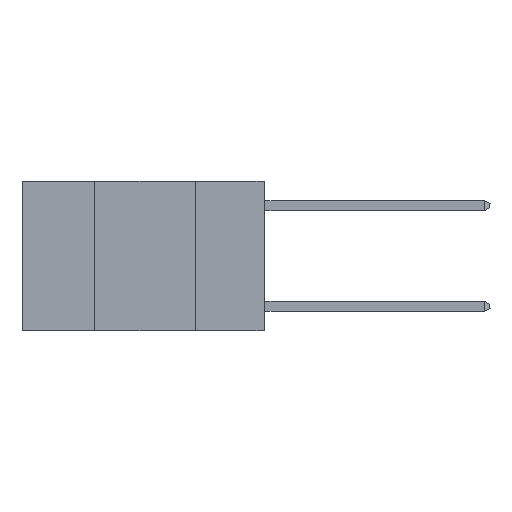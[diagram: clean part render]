
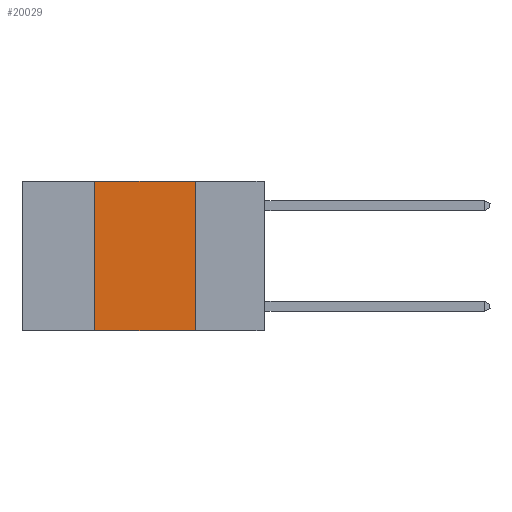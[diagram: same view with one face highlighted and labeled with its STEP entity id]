
A CAD part, left-side view. The second image highlights one B-rep face of the part: STEP entity #20029.
In plain terms, the highlighted planar face has unit normal (-1, 0, 0).
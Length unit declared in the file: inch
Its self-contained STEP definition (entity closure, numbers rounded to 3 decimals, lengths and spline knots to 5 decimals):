
#322 = DIRECTION ( 'NONE',  ( 0., 0., -1. ) ) ;
#1117 = DIRECTION ( 'NONE',  ( 0., 0., 1. ) ) ;
#1171 = ORIENTED_EDGE ( 'NONE', *, *, #13035, .F. ) ;
#1600 = VERTEX_POINT ( 'NONE', #6314 ) ;
#1642 = EDGE_LOOP ( 'NONE', ( #16098, #3742, #1171, #13932 ) ) ;
#3742 = ORIENTED_EDGE ( 'NONE', *, *, #10531, .F. ) ;
#4994 = VERTEX_POINT ( 'NONE', #14117 ) ;
#5290 = LINE ( 'NONE', #5651, #12635 ) ;
#5336 = VECTOR ( 'NONE', #1117, 39.37008 ) ;
#5651 = CARTESIAN_POINT ( 'NONE',  ( 0., 0.17, 0. ) ) ;
#6111 = DIRECTION ( 'NONE',  ( 0., -1., 0. ) ) ;
#6314 = CARTESIAN_POINT ( 'NONE',  ( 0., 0.42, 0. ) ) ;
#6850 = CARTESIAN_POINT ( 'NONE',  ( 0., 0.17, -0.37 ) ) ;
#7582 = VERTEX_POINT ( 'NONE', #6850 ) ;
#7647 = LINE ( 'NONE', #18508, #5336 ) ;
#7866 = VECTOR ( 'NONE', #9376, 39.37008 ) ;
#8068 = CARTESIAN_POINT ( 'NONE',  ( 0., 0.17, 0. ) ) ;
#8636 = DIRECTION ( 'NONE',  ( 0., 0., -1. ) ) ;
#9376 = DIRECTION ( 'NONE',  ( 0., -1., 0. ) ) ;
#9666 = CARTESIAN_POINT ( 'NONE',  ( 0., 0.6, -0.37 ) ) ;
#10531 = EDGE_CURVE ( 'NONE', #1600, #18305, #20348, .T. ) ;
#11920 = DIRECTION ( 'NONE',  ( 1., 0., 0. ) ) ;
#12635 = VECTOR ( 'NONE', #322, 39.37008 ) ;
#13035 = EDGE_CURVE ( 'NONE', #4994, #1600, #7647, .T. ) ;
#13107 = EDGE_CURVE ( 'NONE', #4994, #7582, #22304, .T. ) ;
#13246 = VECTOR ( 'NONE', #6111, 39.37008 ) ;
#13932 = ORIENTED_EDGE ( 'NONE', *, *, #13107, .T. ) ;
#14117 = CARTESIAN_POINT ( 'NONE',  ( 0., 0.42, -0.37 ) ) ;
#15916 = FACE_OUTER_BOUND ( 'NONE', #1642, .T. ) ;
#16098 = ORIENTED_EDGE ( 'NONE', *, *, #22188, .F. ) ;
#18305 = VERTEX_POINT ( 'NONE', #8068 ) ;
#18508 = CARTESIAN_POINT ( 'NONE',  ( 0., 0.42, 0. ) ) ;
#18622 = AXIS2_PLACEMENT_3D ( 'NONE', #19367, #11920, #8636 ) ;
#19367 = CARTESIAN_POINT ( 'NONE',  ( 0., 0.6, 0. ) ) ;
#20029 = ADVANCED_FACE ( 'NONE', ( #15916 ), #22808, .F. ) ;
#20247 = CARTESIAN_POINT ( 'NONE',  ( 0., 0.6, 0. ) ) ;
#20348 = LINE ( 'NONE', #20247, #7866 ) ;
#22188 = EDGE_CURVE ( 'NONE', #18305, #7582, #5290, .T. ) ;
#22304 = LINE ( 'NONE', #9666, #13246 ) ;
#22808 = PLANE ( 'NONE',  #18622 ) ;
